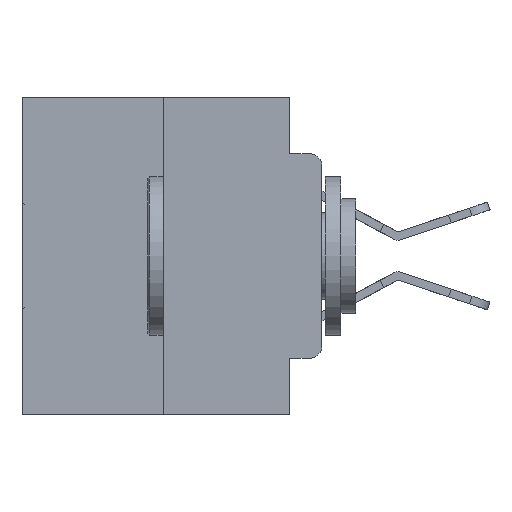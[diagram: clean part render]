
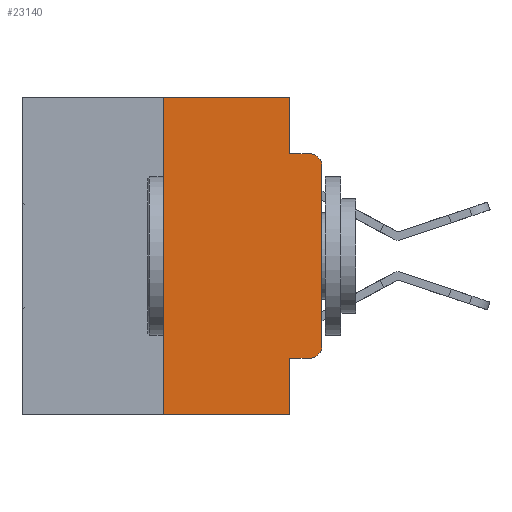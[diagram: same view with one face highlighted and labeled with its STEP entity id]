
A CAD part, left-side view. The second image highlights one B-rep face of the part: STEP entity #23140.
In plain terms, the highlighted planar face has unit normal (-1, 0, 0).
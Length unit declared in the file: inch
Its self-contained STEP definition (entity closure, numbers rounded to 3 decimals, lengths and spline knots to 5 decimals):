
#44 = EDGE_CURVE ( 'NONE', #11498, #12392, #14785, .T. ) ;
#167 = ORIENTED_EDGE ( 'NONE', *, *, #10197, .F. ) ;
#1419 = VERTEX_POINT ( 'NONE', #29127 ) ;
#1785 = VECTOR ( 'NONE', #25490, 39.37008 ) ;
#1865 = CARTESIAN_POINT ( 'NONE',  ( 0., 0.02, -0.0885 ) ) ;
#2180 = VECTOR ( 'NONE', #3960, 39.37008 ) ;
#2399 = VERTEX_POINT ( 'NONE', #15204 ) ;
#2488 = CARTESIAN_POINT ( 'NONE',  ( 0., 0.051, 0. ) ) ;
#3137 = CARTESIAN_POINT ( 'NONE',  ( 0., 0., -0.3915 ) ) ;
#3928 = VERTEX_POINT ( 'NONE', #28449 ) ;
#3960 = DIRECTION ( 'NONE',  ( 0., -1., 0. ) ) ;
#4181 = AXIS2_PLACEMENT_3D ( 'NONE', #12740, #29231, #15131 ) ;
#4875 = VECTOR ( 'NONE', #9671, 39.37008 ) ;
#5640 = LINE ( 'NONE', #9629, #19057 ) ;
#6133 = EDGE_CURVE ( 'NONE', #16707, #28079, #14055, .T. ) ;
#6296 = ORIENTED_EDGE ( 'NONE', *, *, #16223, .T. ) ;
#6312 = CARTESIAN_POINT ( 'NONE',  ( 0., 0.25, 0. ) ) ;
#7507 = CARTESIAN_POINT ( 'NONE',  ( 0., 0.473, 0. ) ) ;
#8541 = DIRECTION ( 'NONE',  ( -1., 0., 0. ) ) ;
#8955 = DIRECTION ( 'NONE',  ( 0., 0., 1. ) ) ;
#8958 = CARTESIAN_POINT ( 'NONE',  ( 0., 0.051, -0.0885 ) ) ;
#9629 = CARTESIAN_POINT ( 'NONE',  ( 0., 0.051, 0. ) ) ;
#9671 = DIRECTION ( 'NONE',  ( 0., 0., -1. ) ) ;
#9800 = CARTESIAN_POINT ( 'NONE',  ( 0., 0.25, -0.5 ) ) ;
#9933 = PLANE ( 'NONE',  #15577 ) ;
#10197 = EDGE_CURVE ( 'NONE', #2399, #12392, #23913, .T. ) ;
#10545 = EDGE_CURVE ( 'NONE', #11845, #3928, #27556, .T. ) ;
#10584 = LINE ( 'NONE', #25045, #27958 ) ;
#11144 = CARTESIAN_POINT ( 'NONE',  ( 0., 0.473, 0. ) ) ;
#11498 = VERTEX_POINT ( 'NONE', #9800 ) ;
#11845 = VERTEX_POINT ( 'NONE', #6312 ) ;
#12250 = AXIS2_PLACEMENT_3D ( 'NONE', #22784, #8541, #25184 ) ;
#12330 = DIRECTION ( 'NONE',  ( 0., 0., -1. ) ) ;
#12392 = VERTEX_POINT ( 'NONE', #20618 ) ;
#12740 = CARTESIAN_POINT ( 'NONE',  ( 0., 0.02, -0.1085 ) ) ;
#13007 = VECTOR ( 'NONE', #8955, 39.37008 ) ;
#13744 = LINE ( 'NONE', #18392, #13007 ) ;
#14055 = CIRCLE ( 'NONE', #4181, 0.02 ) ;
#14285 = LINE ( 'NONE', #21616, #26878 ) ;
#14785 = LINE ( 'NONE', #16777, #21074 ) ;
#15131 = DIRECTION ( 'NONE',  ( 0., 0., -1. ) ) ;
#15204 = CARTESIAN_POINT ( 'NONE',  ( 0., 0.051, -0.4115 ) ) ;
#15577 = AXIS2_PLACEMENT_3D ( 'NONE', #7507, #26536, #12330 ) ;
#16223 = EDGE_CURVE ( 'NONE', #19868, #18826, #17454, .T. ) ;
#16337 = EDGE_CURVE ( 'NONE', #18826, #16707, #13744, .T. ) ;
#16707 = VERTEX_POINT ( 'NONE', #19922 ) ;
#16777 = CARTESIAN_POINT ( 'NONE',  ( 0., 0.473, -0.5 ) ) ;
#17454 = CIRCLE ( 'NONE', #12250, 0.02 ) ;
#17854 = ORIENTED_EDGE ( 'NONE', *, *, #44, .T. ) ;
#18392 = CARTESIAN_POINT ( 'NONE',  ( 0., 0., 0. ) ) ;
#18826 = VERTEX_POINT ( 'NONE', #3137 ) ;
#18930 = ORIENTED_EDGE ( 'NONE', *, *, #16337, .T. ) ;
#19057 = VECTOR ( 'NONE', #26249, 39.37008 ) ;
#19237 = DIRECTION ( 'NONE',  ( 0., -1., 0. ) ) ;
#19673 = ORIENTED_EDGE ( 'NONE', *, *, #6133, .T. ) ;
#19763 = EDGE_LOOP ( 'NONE', ( #18930, #19673, #26025, #21190, #27474, #22694, #17854, #167, #30749, #6296 ) ) ;
#19868 = VERTEX_POINT ( 'NONE', #23961 ) ;
#19922 = CARTESIAN_POINT ( 'NONE',  ( 0., 0., -0.1085 ) ) ;
#20618 = CARTESIAN_POINT ( 'NONE',  ( 0., 0.051, -0.5 ) ) ;
#20889 = LINE ( 'NONE', #8958, #1785 ) ;
#21074 = VECTOR ( 'NONE', #19237, 39.37008 ) ;
#21190 = ORIENTED_EDGE ( 'NONE', *, *, #29380, .F. ) ;
#21391 = FACE_OUTER_BOUND ( 'NONE', #19763, .T. ) ;
#21616 = CARTESIAN_POINT ( 'NONE',  ( 0., 0.25, 0. ) ) ;
#22694 = ORIENTED_EDGE ( 'NONE', *, *, #24116, .F. ) ;
#22784 = CARTESIAN_POINT ( 'NONE',  ( 0., 0.02, -0.3915 ) ) ;
#23140 = ADVANCED_FACE ( 'NONE', ( #21391 ), #9933, .F. ) ;
#23913 = LINE ( 'NONE', #2488, #4875 ) ;
#23961 = CARTESIAN_POINT ( 'NONE',  ( 0., 0.02, -0.4115 ) ) ;
#24116 = EDGE_CURVE ( 'NONE', #11498, #11845, #14285, .T. ) ;
#25045 = CARTESIAN_POINT ( 'NONE',  ( 0., 0.051, -0.4115 ) ) ;
#25184 = DIRECTION ( 'NONE',  ( 0., 0., -1. ) ) ;
#25490 = DIRECTION ( 'NONE',  ( 0., -1., 0. ) ) ;
#26025 = ORIENTED_EDGE ( 'NONE', *, *, #29949, .F. ) ;
#26249 = DIRECTION ( 'NONE',  ( 0., 0., -1. ) ) ;
#26271 = DIRECTION ( 'NONE',  ( 0., 0., 1. ) ) ;
#26536 = DIRECTION ( 'NONE',  ( 1., 0., 0. ) ) ;
#26878 = VECTOR ( 'NONE', #26271, 39.37008 ) ;
#27378 = DIRECTION ( 'NONE',  ( 0., -1., 0. ) ) ;
#27474 = ORIENTED_EDGE ( 'NONE', *, *, #10545, .F. ) ;
#27556 = LINE ( 'NONE', #11144, #2180 ) ;
#27958 = VECTOR ( 'NONE', #27378, 39.37008 ) ;
#28079 = VERTEX_POINT ( 'NONE', #1865 ) ;
#28449 = CARTESIAN_POINT ( 'NONE',  ( 0., 0.051, 0. ) ) ;
#29029 = EDGE_CURVE ( 'NONE', #2399, #19868, #10584, .T. ) ;
#29127 = CARTESIAN_POINT ( 'NONE',  ( 0., 0.051, -0.0885 ) ) ;
#29231 = DIRECTION ( 'NONE',  ( -1., 0., 0. ) ) ;
#29380 = EDGE_CURVE ( 'NONE', #3928, #1419, #5640, .T. ) ;
#29949 = EDGE_CURVE ( 'NONE', #1419, #28079, #20889, .T. ) ;
#30749 = ORIENTED_EDGE ( 'NONE', *, *, #29029, .T. ) ;
